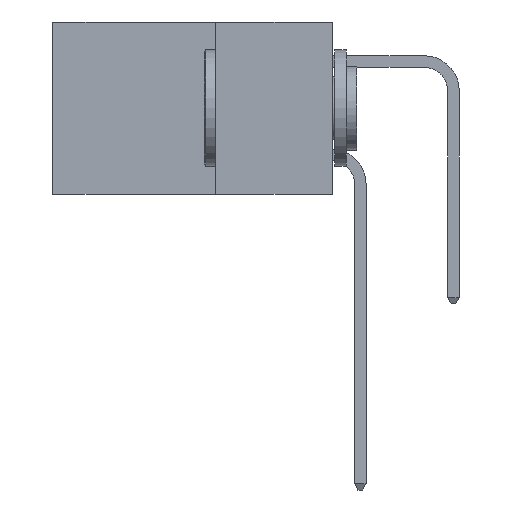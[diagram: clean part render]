
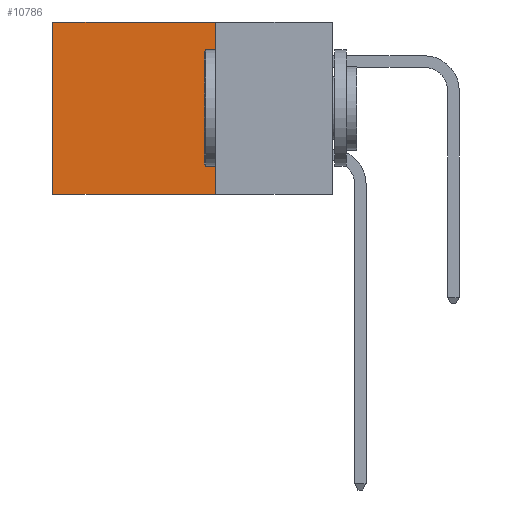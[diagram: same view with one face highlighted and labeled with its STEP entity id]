
A CAD part, left-side view. The second image highlights one B-rep face of the part: STEP entity #10786.
In plain terms, the highlighted planar face has unit normal (-1, 0, 0).
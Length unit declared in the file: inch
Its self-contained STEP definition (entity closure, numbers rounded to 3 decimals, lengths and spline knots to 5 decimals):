
#232 = EDGE_CURVE ( 'NONE', #8858, #15478, #14890, .T. ) ;
#389 = CARTESIAN_POINT ( 'NONE',  ( 0.2615, 0.25, 0. ) ) ;
#439 = EDGE_CURVE ( 'NONE', #12740, #8858, #17315, .T. ) ;
#840 = CARTESIAN_POINT ( 'NONE',  ( 0.2615, 0.25, -0.37 ) ) ;
#1468 = VECTOR ( 'NONE', #13216, 39.37008 ) ;
#1485 = EDGE_CURVE ( 'NONE', #12740, #10632, #6752, .T. ) ;
#1731 = DIRECTION ( 'NONE',  ( 0., 0., -1. ) ) ;
#2703 = CARTESIAN_POINT ( 'NONE',  ( 0.2615, 0.25, -0.37 ) ) ;
#5173 = EDGE_CURVE ( 'NONE', #10632, #15478, #5262, .T. ) ;
#5262 = LINE ( 'NONE', #13334, #1468 ) ;
#5292 = DIRECTION ( 'NONE',  ( 0., 1., 0. ) ) ;
#5680 = CARTESIAN_POINT ( 'NONE',  ( 0.2615, 0.25, 0. ) ) ;
#6752 = LINE ( 'NONE', #5680, #13941 ) ;
#7173 = ORIENTED_EDGE ( 'NONE', *, *, #232, .F. ) ;
#8858 = VERTEX_POINT ( 'NONE', #2703 ) ;
#9988 = VECTOR ( 'NONE', #1731, 39.37008 ) ;
#10632 = VERTEX_POINT ( 'NONE', #13341 ) ;
#10773 = FACE_OUTER_BOUND ( 'NONE', #11051, .T. ) ;
#10786 = ADVANCED_FACE ( 'NONE', ( #10773 ), #12101, .F. ) ;
#10845 = ORIENTED_EDGE ( 'NONE', *, *, #439, .F. ) ;
#11051 = EDGE_LOOP ( 'NONE', ( #12725, #7173, #10845, #14309 ) ) ;
#11880 = DIRECTION ( 'NONE',  ( 0., 0., -1. ) ) ;
#11906 = DIRECTION ( 'NONE',  ( 1., 0., 0. ) ) ;
#11921 = CARTESIAN_POINT ( 'NONE',  ( 0.2615, 0.25, -0.37 ) ) ;
#12101 = PLANE ( 'NONE',  #13207 ) ;
#12725 = ORIENTED_EDGE ( 'NONE', *, *, #5173, .T. ) ;
#12740 = VERTEX_POINT ( 'NONE', #389 ) ;
#13207 = AXIS2_PLACEMENT_3D ( 'NONE', #11921, #11906, #11880 ) ;
#13216 = DIRECTION ( 'NONE',  ( 0., 0., -1. ) ) ;
#13334 = CARTESIAN_POINT ( 'NONE',  ( 0.2615, 0.6, -0.37 ) ) ;
#13341 = CARTESIAN_POINT ( 'NONE',  ( 0.2615, 0.6, 0. ) ) ;
#13941 = VECTOR ( 'NONE', #15760, 39.37008 ) ;
#14309 = ORIENTED_EDGE ( 'NONE', *, *, #1485, .T. ) ;
#14890 = LINE ( 'NONE', #840, #16732 ) ;
#15072 = CARTESIAN_POINT ( 'NONE',  ( 0.2615, 0.6, -0.37 ) ) ;
#15478 = VERTEX_POINT ( 'NONE', #15072 ) ;
#15760 = DIRECTION ( 'NONE',  ( 0., 1., 0. ) ) ;
#16732 = VECTOR ( 'NONE', #5292, 39.37008 ) ;
#17315 = LINE ( 'NONE', #17515, #9988 ) ;
#17515 = CARTESIAN_POINT ( 'NONE',  ( 0.2615, 0.25, -0.37 ) ) ;
